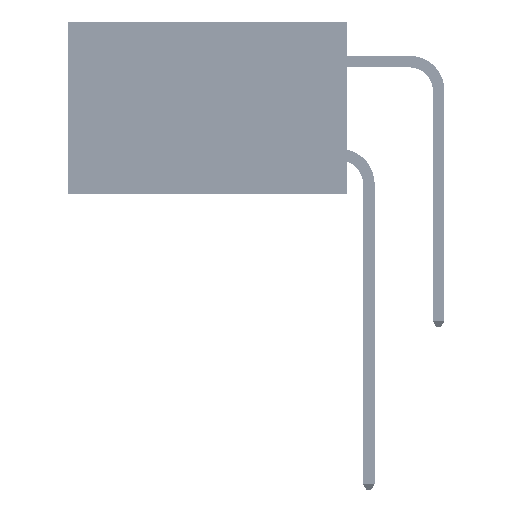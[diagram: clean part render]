
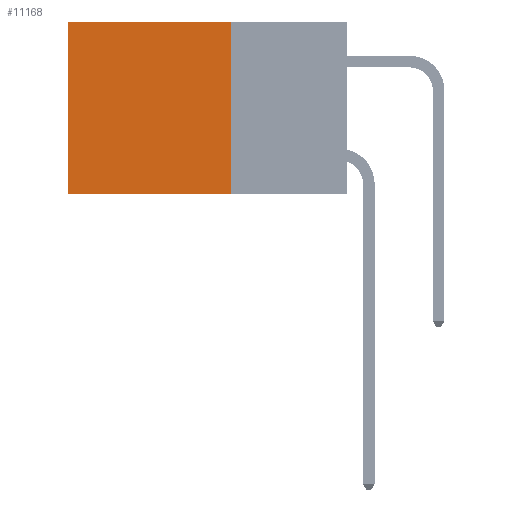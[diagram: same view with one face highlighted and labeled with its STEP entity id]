
A CAD part, left-side view. The second image highlights one B-rep face of the part: STEP entity #11168.
In plain terms, the highlighted planar face has unit normal (-1, 0, 0).
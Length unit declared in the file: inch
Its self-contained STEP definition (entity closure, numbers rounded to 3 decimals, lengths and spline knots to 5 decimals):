
#293 = CARTESIAN_POINT ( 'NONE',  ( 0.2875, 0.6, 0. ) ) ;
#1913 = CARTESIAN_POINT ( 'NONE',  ( 0.2875, 0.6, 0. ) ) ;
#3929 = DIRECTION ( 'NONE',  ( 0., 0., -1. ) ) ;
#4011 = DIRECTION ( 'NONE',  ( 0., 0., -1. ) ) ;
#7514 = EDGE_CURVE ( 'NONE', #7583, #24552, #37737, .T. ) ;
#7583 = VERTEX_POINT ( 'NONE', #7986 ) ;
#7986 = CARTESIAN_POINT ( 'NONE',  ( 0.2875, 0.25, 0. ) ) ;
#8925 = CARTESIAN_POINT ( 'NONE',  ( 0.2875, 0.25, 0. ) ) ;
#10049 = LINE ( 'NONE', #8925, #17450 ) ;
#11168 = ADVANCED_FACE ( 'NONE', ( #29480 ), #25798, .F. ) ;
#13751 = LINE ( 'NONE', #293, #16625 ) ;
#15556 = ORIENTED_EDGE ( 'NONE', *, *, #28709, .F. ) ;
#16125 = EDGE_CURVE ( 'NONE', #24552, #21264, #13751, .T. ) ;
#16333 = CARTESIAN_POINT ( 'NONE',  ( 0.2875, 0.25, -0.37 ) ) ;
#16625 = VECTOR ( 'NONE', #3929, 39.37008 ) ;
#17450 = VECTOR ( 'NONE', #41688, 39.37008 ) ;
#17639 = CARTESIAN_POINT ( 'NONE',  ( 0.2875, 0.6, -0.37 ) ) ;
#18710 = ORIENTED_EDGE ( 'NONE', *, *, #33159, .F. ) ;
#21264 = VERTEX_POINT ( 'NONE', #17639 ) ;
#23609 = EDGE_LOOP ( 'NONE', ( #23820, #15556, #18710, #24629 ) ) ;
#23820 = ORIENTED_EDGE ( 'NONE', *, *, #16125, .T. ) ;
#24348 = DIRECTION ( 'NONE',  ( 0., 1., 0. ) ) ;
#24552 = VERTEX_POINT ( 'NONE', #1913 ) ;
#24629 = ORIENTED_EDGE ( 'NONE', *, *, #7514, .T. ) ;
#25798 = PLANE ( 'NONE',  #45056 ) ;
#28709 = EDGE_CURVE ( 'NONE', #29685, #21264, #43562, .T. ) ;
#29480 = FACE_OUTER_BOUND ( 'NONE', #23609, .T. ) ;
#29685 = VERTEX_POINT ( 'NONE', #16333 ) ;
#32778 = VECTOR ( 'NONE', #24348, 39.37008 ) ;
#33159 = EDGE_CURVE ( 'NONE', #7583, #29685, #10049, .T. ) ;
#33476 = DIRECTION ( 'NONE',  ( 1., 0., 0. ) ) ;
#35212 = CARTESIAN_POINT ( 'NONE',  ( 0.2875, 0.25, -0.37 ) ) ;
#36807 = CARTESIAN_POINT ( 'NONE',  ( 0.2875, 0.25, 0. ) ) ;
#37737 = LINE ( 'NONE', #44417, #45114 ) ;
#40603 = DIRECTION ( 'NONE',  ( 0., 1., 0. ) ) ;
#41688 = DIRECTION ( 'NONE',  ( 0., 0., -1. ) ) ;
#43562 = LINE ( 'NONE', #35212, #32778 ) ;
#44417 = CARTESIAN_POINT ( 'NONE',  ( 0.2875, 0.25, 0. ) ) ;
#45056 = AXIS2_PLACEMENT_3D ( 'NONE', #36807, #33476, #4011 ) ;
#45114 = VECTOR ( 'NONE', #40603, 39.37008 ) ;
